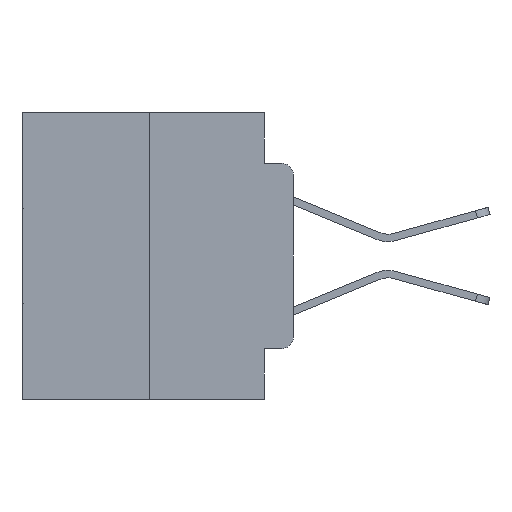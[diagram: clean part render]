
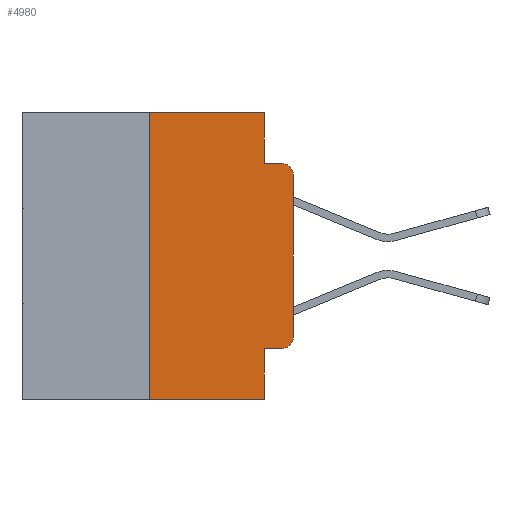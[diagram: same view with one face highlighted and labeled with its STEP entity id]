
A CAD part, left-side view. The second image highlights one B-rep face of the part: STEP entity #4980.
In plain terms, the highlighted planar face has unit normal (-1, 0, 0).
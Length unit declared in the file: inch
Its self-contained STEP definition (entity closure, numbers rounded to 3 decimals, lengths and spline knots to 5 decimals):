
#23 = DIRECTION ( 'NONE',  ( 0., 0., 1. ) ) ;
#73 = DIRECTION ( 'NONE',  ( 0., 0., 1. ) ) ;
#1237 = ORIENTED_EDGE ( 'NONE', *, *, #20879, .F. ) ;
#1261 = FACE_OUTER_BOUND ( 'NONE', #4438, .T. ) ;
#1382 = EDGE_CURVE ( 'NONE', #2092, #3688, #20147, .T. ) ;
#2092 = VERTEX_POINT ( 'NONE', #14827 ) ;
#2117 = EDGE_CURVE ( 'NONE', #18256, #14894, #2241, .T. ) ;
#2175 = LINE ( 'NONE', #19657, #16167 ) ;
#2241 = LINE ( 'NONE', #4675, #24273 ) ;
#2363 = LINE ( 'NONE', #26235, #20822 ) ;
#2677 = DIRECTION ( 'NONE',  ( 0., 0., -1. ) ) ;
#2738 = ORIENTED_EDGE ( 'NONE', *, *, #1382, .T. ) ;
#2974 = VERTEX_POINT ( 'NONE', #23618 ) ;
#2995 = CARTESIAN_POINT ( 'NONE',  ( 0., 0.473, 0. ) ) ;
#3364 = CARTESIAN_POINT ( 'NONE',  ( 0., 0., -0.3915 ) ) ;
#3688 = VERTEX_POINT ( 'NONE', #3364 ) ;
#4321 = ORIENTED_EDGE ( 'NONE', *, *, #25619, .T. ) ;
#4410 = EDGE_CURVE ( 'NONE', #5344, #26466, #2175, .T. ) ;
#4438 = EDGE_LOOP ( 'NONE', ( #4321, #26772, #1237, #26047, #15413, #28222, #22489, #22259, #11466, #2738 ) ) ;
#4675 = CARTESIAN_POINT ( 'NONE',  ( 0., 0.051, 0. ) ) ;
#4980 = ADVANCED_FACE ( 'NONE', ( #1261 ), #9976, .F. ) ;
#5310 = LINE ( 'NONE', #22923, #15848 ) ;
#5344 = VERTEX_POINT ( 'NONE', #16130 ) ;
#5359 = LINE ( 'NONE', #7907, #21722 ) ;
#5670 = CARTESIAN_POINT ( 'NONE',  ( 0., 0.051, -0.0885 ) ) ;
#7176 = AXIS2_PLACEMENT_3D ( 'NONE', #26691, #10203, #2677 ) ;
#7735 = VECTOR ( 'NONE', #15503, 39.37008 ) ;
#7907 = CARTESIAN_POINT ( 'NONE',  ( 0., 0.051, -0.4115 ) ) ;
#8264 = VECTOR ( 'NONE', #21546, 39.37008 ) ;
#8467 = VERTEX_POINT ( 'NONE', #5670 ) ;
#8745 = VECTOR ( 'NONE', #20556, 39.37008 ) ;
#9281 = DIRECTION ( 'NONE',  ( -1., 0., 0. ) ) ;
#9614 = CARTESIAN_POINT ( 'NONE',  ( 0., 0.051, -0.4115 ) ) ;
#9776 = EDGE_CURVE ( 'NONE', #26883, #8467, #12789, .T. ) ;
#9976 = PLANE ( 'NONE',  #23080 ) ;
#10203 = DIRECTION ( 'NONE',  ( -1., 0., 0. ) ) ;
#10375 = CIRCLE ( 'NONE', #7176, 0.02 ) ;
#11020 = CARTESIAN_POINT ( 'NONE',  ( 0., 0.02, -0.3915 ) ) ;
#11466 = ORIENTED_EDGE ( 'NONE', *, *, #24747, .T. ) ;
#12152 = DIRECTION ( 'NONE',  ( 0., -1., 0. ) ) ;
#12334 = DIRECTION ( 'NONE',  ( 0., -1., 0. ) ) ;
#12789 = LINE ( 'NONE', #26054, #8264 ) ;
#12815 = AXIS2_PLACEMENT_3D ( 'NONE', #11020, #9281, #13588 ) ;
#13588 = DIRECTION ( 'NONE',  ( 0., 0., -1. ) ) ;
#14404 = CARTESIAN_POINT ( 'NONE',  ( 0., 0.051, 0. ) ) ;
#14688 = EDGE_CURVE ( 'NONE', #5344, #14894, #5310, .T. ) ;
#14827 = CARTESIAN_POINT ( 'NONE',  ( 0., 0.02, -0.4115 ) ) ;
#14894 = VERTEX_POINT ( 'NONE', #16923 ) ;
#15413 = ORIENTED_EDGE ( 'NONE', *, *, #18022, .F. ) ;
#15503 = DIRECTION ( 'NONE',  ( 0., -1., 0. ) ) ;
#15848 = VECTOR ( 'NONE', #12152, 39.37008 ) ;
#16130 = CARTESIAN_POINT ( 'NONE',  ( 0., 0.25, -0.5 ) ) ;
#16167 = VECTOR ( 'NONE', #23, 39.37008 ) ;
#16570 = CARTESIAN_POINT ( 'NONE',  ( 0., 0.051, -0.0885 ) ) ;
#16923 = CARTESIAN_POINT ( 'NONE',  ( 0., 0.051, -0.5 ) ) ;
#17154 = LINE ( 'NONE', #21860, #7735 ) ;
#18022 = EDGE_CURVE ( 'NONE', #26466, #26883, #17154, .T. ) ;
#18256 = VERTEX_POINT ( 'NONE', #9614 ) ;
#18747 = DIRECTION ( 'NONE',  ( 1., 0., 0. ) ) ;
#19657 = CARTESIAN_POINT ( 'NONE',  ( 0., 0.25, 0. ) ) ;
#19698 = CARTESIAN_POINT ( 'NONE',  ( 0., 0.02, -0.0885 ) ) ;
#20147 = CIRCLE ( 'NONE', #12815, 0.02 ) ;
#20556 = DIRECTION ( 'NONE',  ( 0., -1., 0. ) ) ;
#20822 = VECTOR ( 'NONE', #73, 39.37008 ) ;
#20879 = EDGE_CURVE ( 'NONE', #8467, #24404, #22867, .T. ) ;
#21546 = DIRECTION ( 'NONE',  ( 0., 0., -1. ) ) ;
#21722 = VECTOR ( 'NONE', #12334, 39.37008 ) ;
#21860 = CARTESIAN_POINT ( 'NONE',  ( 0., 0.473, 0. ) ) ;
#22259 = ORIENTED_EDGE ( 'NONE', *, *, #2117, .F. ) ;
#22489 = ORIENTED_EDGE ( 'NONE', *, *, #14688, .T. ) ;
#22867 = LINE ( 'NONE', #16570, #8745 ) ;
#22923 = CARTESIAN_POINT ( 'NONE',  ( 0., 0.473, -0.5 ) ) ;
#23080 = AXIS2_PLACEMENT_3D ( 'NONE', #2995, #18747, #24730 ) ;
#23618 = CARTESIAN_POINT ( 'NONE',  ( 0., 0., -0.1085 ) ) ;
#24273 = VECTOR ( 'NONE', #26678, 39.37008 ) ;
#24404 = VERTEX_POINT ( 'NONE', #19698 ) ;
#24730 = DIRECTION ( 'NONE',  ( 0., 0., -1. ) ) ;
#24747 = EDGE_CURVE ( 'NONE', #18256, #2092, #5359, .T. ) ;
#25619 = EDGE_CURVE ( 'NONE', #3688, #2974, #2363, .T. ) ;
#26047 = ORIENTED_EDGE ( 'NONE', *, *, #9776, .F. ) ;
#26054 = CARTESIAN_POINT ( 'NONE',  ( 0., 0.051, 0. ) ) ;
#26235 = CARTESIAN_POINT ( 'NONE',  ( 0., 0., 0. ) ) ;
#26466 = VERTEX_POINT ( 'NONE', #27028 ) ;
#26678 = DIRECTION ( 'NONE',  ( 0., 0., -1. ) ) ;
#26691 = CARTESIAN_POINT ( 'NONE',  ( 0., 0.02, -0.1085 ) ) ;
#26772 = ORIENTED_EDGE ( 'NONE', *, *, #27208, .T. ) ;
#26883 = VERTEX_POINT ( 'NONE', #14404 ) ;
#27028 = CARTESIAN_POINT ( 'NONE',  ( 0., 0.25, 0. ) ) ;
#27208 = EDGE_CURVE ( 'NONE', #2974, #24404, #10375, .T. ) ;
#28222 = ORIENTED_EDGE ( 'NONE', *, *, #4410, .F. ) ;
